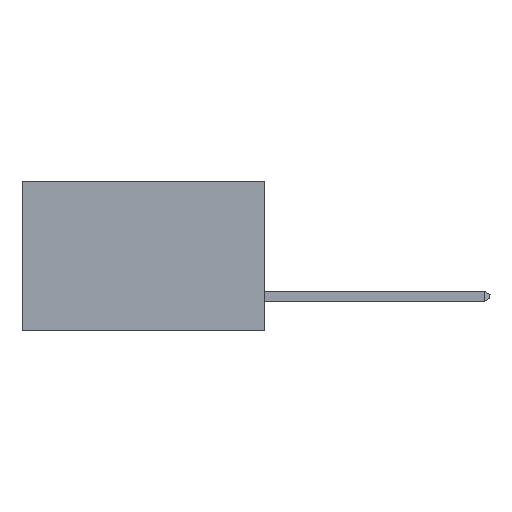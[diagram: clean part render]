
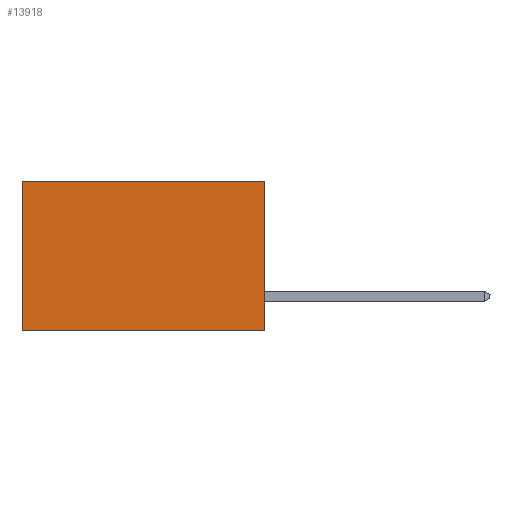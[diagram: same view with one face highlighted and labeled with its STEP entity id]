
A CAD part, left-side view. The second image highlights one B-rep face of the part: STEP entity #13918.
In plain terms, the highlighted planar face has unit normal (-1, 0, 0).
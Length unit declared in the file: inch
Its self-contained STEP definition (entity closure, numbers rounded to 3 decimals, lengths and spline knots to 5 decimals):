
#86 = CARTESIAN_POINT ( 'NONE',  ( 0.298, 0.6, 0. ) ) ;
#163 = VERTEX_POINT ( 'NONE', #597 ) ;
#597 = CARTESIAN_POINT ( 'NONE',  ( 0.298, 0., 0. ) ) ;
#1741 = DIRECTION ( 'NONE',  ( 0., 0., -1. ) ) ;
#1893 = EDGE_CURVE ( 'NONE', #163, #6384, #2500, .T. ) ;
#2211 = CARTESIAN_POINT ( 'NONE',  ( 0.298, 0., -0.37 ) ) ;
#2457 = CARTESIAN_POINT ( 'NONE',  ( 0.298, 0., 0. ) ) ;
#2500 = LINE ( 'NONE', #22992, #14958 ) ;
#2628 = DIRECTION ( 'NONE',  ( 0., 1., 0. ) ) ;
#3178 = EDGE_CURVE ( 'NONE', #6384, #5529, #12389, .T. ) ;
#3680 = PLANE ( 'NONE',  #12275 ) ;
#3976 = EDGE_CURVE ( 'NONE', #163, #10603, #19825, .T. ) ;
#5529 = VERTEX_POINT ( 'NONE', #8689 ) ;
#6384 = VERTEX_POINT ( 'NONE', #2211 ) ;
#6957 = ORIENTED_EDGE ( 'NONE', *, *, #10712, .T. ) ;
#6979 = VECTOR ( 'NONE', #1741, 39.37008 ) ;
#7141 = FACE_OUTER_BOUND ( 'NONE', #10834, .T. ) ;
#8689 = CARTESIAN_POINT ( 'NONE',  ( 0.298, 0.6, -0.37 ) ) ;
#9553 = VECTOR ( 'NONE', #19802, 39.37008 ) ;
#10603 = VERTEX_POINT ( 'NONE', #15516 ) ;
#10712 = EDGE_CURVE ( 'NONE', #10603, #5529, #16958, .T. ) ;
#10834 = EDGE_LOOP ( 'NONE', ( #6957, #18856, #19063, #11439 ) ) ;
#11439 = ORIENTED_EDGE ( 'NONE', *, *, #3976, .T. ) ;
#12035 = DIRECTION ( 'NONE',  ( 0., 0., -1. ) ) ;
#12094 = VECTOR ( 'NONE', #2628, 39.37008 ) ;
#12275 = AXIS2_PLACEMENT_3D ( 'NONE', #14102, #17765, #15898 ) ;
#12389 = LINE ( 'NONE', #13224, #12094 ) ;
#13224 = CARTESIAN_POINT ( 'NONE',  ( 0.298, 0., -0.37 ) ) ;
#13918 = ADVANCED_FACE ( 'NONE', ( #7141 ), #3680, .F. ) ;
#14102 = CARTESIAN_POINT ( 'NONE',  ( 0.298, 0., 0. ) ) ;
#14958 = VECTOR ( 'NONE', #12035, 39.37008 ) ;
#15516 = CARTESIAN_POINT ( 'NONE',  ( 0.298, 0.6, 0. ) ) ;
#15898 = DIRECTION ( 'NONE',  ( 0., 0., -1. ) ) ;
#16958 = LINE ( 'NONE', #86, #6979 ) ;
#17765 = DIRECTION ( 'NONE',  ( 1., 0., 0. ) ) ;
#18856 = ORIENTED_EDGE ( 'NONE', *, *, #3178, .F. ) ;
#19063 = ORIENTED_EDGE ( 'NONE', *, *, #1893, .F. ) ;
#19802 = DIRECTION ( 'NONE',  ( 0., 1., 0. ) ) ;
#19825 = LINE ( 'NONE', #2457, #9553 ) ;
#22992 = CARTESIAN_POINT ( 'NONE',  ( 0.298, 0., 0. ) ) ;
